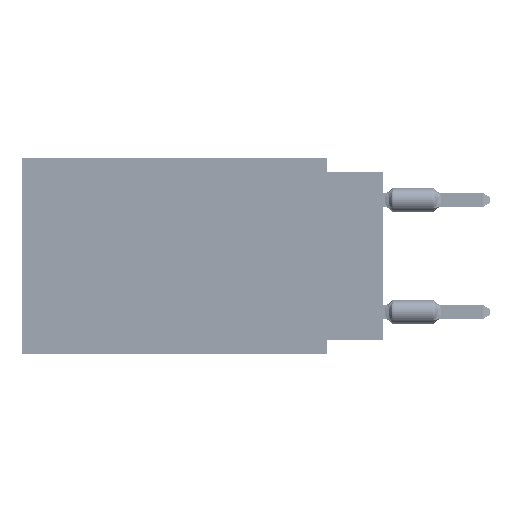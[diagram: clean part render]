
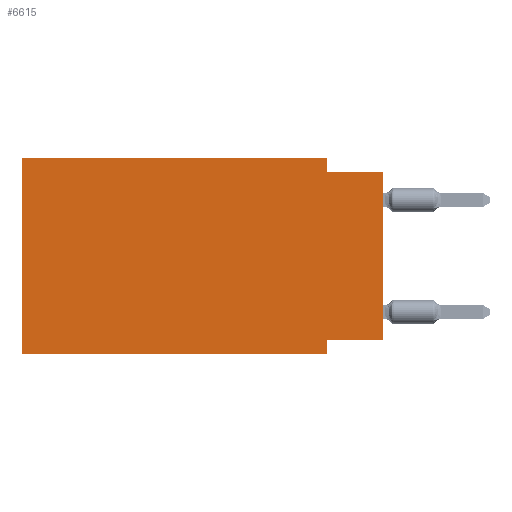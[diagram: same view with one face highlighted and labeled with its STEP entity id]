
A CAD part, left-side view. The second image highlights one B-rep face of the part: STEP entity #6615.
In plain terms, the highlighted planar face has unit normal (-1, 0, 0).
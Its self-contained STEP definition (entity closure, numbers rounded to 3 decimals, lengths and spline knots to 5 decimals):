
#63 = LINE ( 'NONE', #84134, #65454 ) ;
#2484 = CARTESIAN_POINT ( 'NONE',  ( 0., 0.1, 0. ) ) ;
#4569 = PLANE ( 'NONE',  #64747 ) ;
#5131 = VERTEX_POINT ( 'NONE', #16755 ) ;
#5709 = CARTESIAN_POINT ( 'NONE',  ( 0., 0.1, -0.35 ) ) ;
#6086 = DIRECTION ( 'NONE',  ( 1., 0., 0. ) ) ;
#6615 = ADVANCED_FACE ( 'NONE', ( #12668 ), #4569, .F. ) ;
#12668 = FACE_OUTER_BOUND ( 'NONE', #35292, .T. ) ;
#14081 = ORIENTED_EDGE ( 'NONE', *, *, #74300, .T. ) ;
#16755 = CARTESIAN_POINT ( 'NONE',  ( 0., 0., -0.325 ) ) ;
#18922 = CARTESIAN_POINT ( 'NONE',  ( 0., 0.1, -0.325 ) ) ;
#19574 = DIRECTION ( 'NONE',  ( 0., -1., 0. ) ) ;
#21120 = DIRECTION ( 'NONE',  ( 0., -1., 0. ) ) ;
#24370 = VECTOR ( 'NONE', #46746, 39.37008 ) ;
#24536 = EDGE_CURVE ( 'NONE', #83742, #67760, #99361, .T. ) ;
#35292 = EDGE_LOOP ( 'NONE', ( #14081, #79735, #41804, #96035, #70026, #85472, #68169, #72235 ) ) ;
#35629 = LINE ( 'NONE', #50812, #48402 ) ;
#36420 = EDGE_CURVE ( 'NONE', #76346, #71537, #83909, .T. ) ;
#37747 = LINE ( 'NONE', #99554, #47637 ) ;
#38539 = VERTEX_POINT ( 'NONE', #59379 ) ;
#38979 = CARTESIAN_POINT ( 'NONE',  ( 0., 0.1, -0.35 ) ) ;
#41804 = ORIENTED_EDGE ( 'NONE', *, *, #58611, .F. ) ;
#46746 = DIRECTION ( 'NONE',  ( 0., -1., 0. ) ) ;
#47637 = VECTOR ( 'NONE', #61044, 39.37008 ) ;
#47967 = EDGE_CURVE ( 'NONE', #77479, #76346, #63, .T. ) ;
#48223 = CARTESIAN_POINT ( 'NONE',  ( 0., 0., -0.025 ) ) ;
#48402 = VECTOR ( 'NONE', #81734, 39.37008 ) ;
#50812 = CARTESIAN_POINT ( 'NONE',  ( 0., 0.1, 0. ) ) ;
#58611 = EDGE_CURVE ( 'NONE', #71537, #38539, #35629, .T. ) ;
#59379 = CARTESIAN_POINT ( 'NONE',  ( 0., 0.1, -0.025 ) ) ;
#60856 = DIRECTION ( 'NONE',  ( 0., 0., -1. ) ) ;
#61044 = DIRECTION ( 'NONE',  ( 0., 1., 0. ) ) ;
#62320 = LINE ( 'NONE', #77501, #80655 ) ;
#62336 = DIRECTION ( 'NONE',  ( 0., 0., 1. ) ) ;
#63430 = LINE ( 'NONE', #48223, #24370 ) ;
#64747 = AXIS2_PLACEMENT_3D ( 'NONE', #73935, #6086, #98734 ) ;
#65454 = VECTOR ( 'NONE', #62336, 39.37008 ) ;
#65653 = LINE ( 'NONE', #96573, #97880 ) ;
#66663 = CARTESIAN_POINT ( 'NONE',  ( 0., 0.645, -0.35 ) ) ;
#67760 = VERTEX_POINT ( 'NONE', #38979 ) ;
#68169 = ORIENTED_EDGE ( 'NONE', *, *, #24536, .F. ) ;
#69666 = EDGE_CURVE ( 'NONE', #77479, #67760, #65653, .T. ) ;
#70026 = ORIENTED_EDGE ( 'NONE', *, *, #47967, .F. ) ;
#71537 = VERTEX_POINT ( 'NONE', #2484 ) ;
#72235 = ORIENTED_EDGE ( 'NONE', *, *, #84681, .F. ) ;
#72745 = CARTESIAN_POINT ( 'NONE',  ( 0., 0.645, 0. ) ) ;
#73935 = CARTESIAN_POINT ( 'NONE',  ( 0., 0.645, 0. ) ) ;
#74300 = EDGE_CURVE ( 'NONE', #5131, #81780, #62320, .T. ) ;
#76346 = VERTEX_POINT ( 'NONE', #72745 ) ;
#77479 = VERTEX_POINT ( 'NONE', #66663 ) ;
#77501 = CARTESIAN_POINT ( 'NONE',  ( 0., 0., 0. ) ) ;
#78179 = EDGE_CURVE ( 'NONE', #38539, #81780, #63430, .T. ) ;
#78982 = VECTOR ( 'NONE', #60856, 39.37008 ) ;
#79735 = ORIENTED_EDGE ( 'NONE', *, *, #78179, .F. ) ;
#80655 = VECTOR ( 'NONE', #93213, 39.37008 ) ;
#81734 = DIRECTION ( 'NONE',  ( 0., 0., -1. ) ) ;
#81780 = VERTEX_POINT ( 'NONE', #89594 ) ;
#83742 = VERTEX_POINT ( 'NONE', #18922 ) ;
#83909 = LINE ( 'NONE', #84405, #95071 ) ;
#84134 = CARTESIAN_POINT ( 'NONE',  ( 0., 0.645, 0. ) ) ;
#84405 = CARTESIAN_POINT ( 'NONE',  ( 0., 0.645, 0. ) ) ;
#84681 = EDGE_CURVE ( 'NONE', #5131, #83742, #37747, .T. ) ;
#85472 = ORIENTED_EDGE ( 'NONE', *, *, #69666, .T. ) ;
#89594 = CARTESIAN_POINT ( 'NONE',  ( 0., 0., -0.025 ) ) ;
#93213 = DIRECTION ( 'NONE',  ( 0., 0., 1. ) ) ;
#95071 = VECTOR ( 'NONE', #21120, 39.37008 ) ;
#96035 = ORIENTED_EDGE ( 'NONE', *, *, #36420, .F. ) ;
#96573 = CARTESIAN_POINT ( 'NONE',  ( 0., 0.645, -0.35 ) ) ;
#97880 = VECTOR ( 'NONE', #19574, 39.37008 ) ;
#98734 = DIRECTION ( 'NONE',  ( 0., 0., -1. ) ) ;
#99361 = LINE ( 'NONE', #5709, #78982 ) ;
#99554 = CARTESIAN_POINT ( 'NONE',  ( 0., 0., -0.325 ) ) ;
